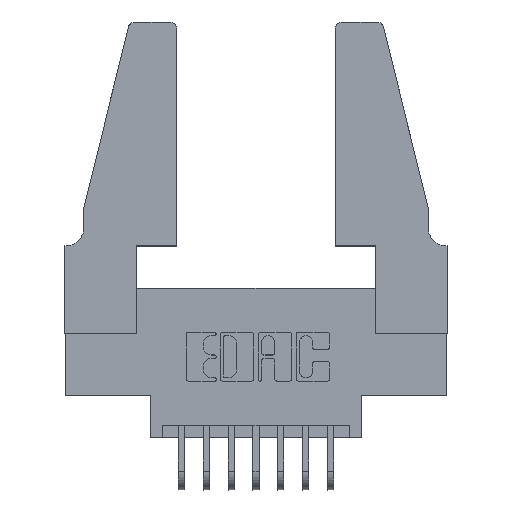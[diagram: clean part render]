
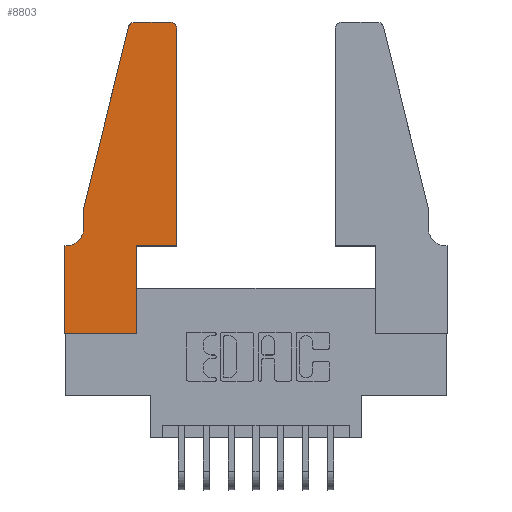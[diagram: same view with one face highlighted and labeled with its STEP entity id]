
A CAD part, top view. The second image highlights one B-rep face of the part: STEP entity #8803.
In plain terms, the highlighted planar face has unit normal (0, 0, 1).
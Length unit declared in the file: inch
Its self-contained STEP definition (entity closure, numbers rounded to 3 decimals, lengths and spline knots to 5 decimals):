
#18 = VECTOR ( 'NONE', #14092, 39.37008 ) ;
#74 = CARTESIAN_POINT ( 'NONE',  ( 0.284, 1.22, 0.37 ) ) ;
#455 = DIRECTION ( 'NONE',  ( 0., 0., 1. ) ) ;
#497 = LINE ( 'NONE', #12305, #11872 ) ;
#555 = CARTESIAN_POINT ( 'NONE',  ( 0.2865, 0., 0.37 ) ) ;
#579 = VERTEX_POINT ( 'NONE', #555 ) ;
#904 = EDGE_CURVE ( 'NONE', #11357, #10992, #4148, .T. ) ;
#951 = EDGE_CURVE ( 'NONE', #3013, #579, #11669, .T. ) ;
#1309 = DIRECTION ( 'NONE',  ( 1., 0., 0. ) ) ;
#1459 = CIRCLE ( 'NONE', #4887, 0.03 ) ;
#1518 = EDGE_CURVE ( 'NONE', #5218, #6235, #2289, .T. ) ;
#1893 = CARTESIAN_POINT ( 'NONE',  ( 0.4205, 1.25, 0.37 ) ) ;
#1919 = VECTOR ( 'NONE', #11491, 39.37008 ) ;
#2080 = CARTESIAN_POINT ( 'NONE',  ( 0.4505, 0.35, 0.37 ) ) ;
#2279 = DIRECTION ( 'NONE',  ( 0., 0., -1. ) ) ;
#2289 = LINE ( 'NONE', #10027, #1919 ) ;
#2444 = CARTESIAN_POINT ( 'NONE',  ( 0., 0.35, 0.37 ) ) ;
#2829 = DIRECTION ( 'NONE',  ( -0.239, -0.971, 0. ) ) ;
#2885 = LINE ( 'NONE', #7581, #8432 ) ;
#3013 = VERTEX_POINT ( 'NONE', #5641 ) ;
#3182 = LINE ( 'NONE', #4582, #18 ) ;
#3295 = VERTEX_POINT ( 'NONE', #8184 ) ;
#3577 = CARTESIAN_POINT ( 'NONE',  ( 0.2865, 0.35, 0.37 ) ) ;
#3605 = DIRECTION ( 'NONE',  ( 1., 0., 0. ) ) ;
#3645 = CARTESIAN_POINT ( 'NONE',  ( 0.0055, 0.35, 0.37 ) ) ;
#3731 = CARTESIAN_POINT ( 'NONE',  ( 0.25487, 1.22718, 0.37 ) ) ;
#4148 = LINE ( 'NONE', #2080, #6389 ) ;
#4316 = CARTESIAN_POINT ( 'NONE',  ( 0.4505, 0.35, 0.37 ) ) ;
#4422 = LINE ( 'NONE', #6341, #12572 ) ;
#4571 = CIRCLE ( 'NONE', #13946, 0.03 ) ;
#4582 = CARTESIAN_POINT ( 'NONE',  ( 0.2605, 1.25, 0.37 ) ) ;
#4646 = LINE ( 'NONE', #3577, #12780 ) ;
#4806 = VERTEX_POINT ( 'NONE', #9488 ) ;
#4812 = CARTESIAN_POINT ( 'NONE',  ( 0.284, 1.25, 0.37 ) ) ;
#4887 = AXIS2_PLACEMENT_3D ( 'NONE', #7293, #455, #8369 ) ;
#5198 = EDGE_CURVE ( 'NONE', #12901, #10067, #4571, .T. ) ;
#5206 = EDGE_LOOP ( 'NONE', ( #6011, #6132, #6167, #6295, #6393, #6473, #6546, #6568, #6668, #6693, #7019, #7049 ) ) ;
#5218 = VERTEX_POINT ( 'NONE', #3645 ) ;
#5641 = CARTESIAN_POINT ( 'NONE',  ( 0., 0., 0.37 ) ) ;
#5981 = EDGE_CURVE ( 'NONE', #10067, #7296, #497, .T. ) ;
#6011 = ORIENTED_EDGE ( 'NONE', *, *, #8704, .T. ) ;
#6132 = ORIENTED_EDGE ( 'NONE', *, *, #5198, .T. ) ;
#6134 = VERTEX_POINT ( 'NONE', #1893 ) ;
#6167 = ORIENTED_EDGE ( 'NONE', *, *, #5981, .T. ) ;
#6235 = VERTEX_POINT ( 'NONE', #11934 ) ;
#6295 = ORIENTED_EDGE ( 'NONE', *, *, #12556, .T. ) ;
#6341 = CARTESIAN_POINT ( 'NONE',  ( 0.4505, 0.35, 0.37 ) ) ;
#6389 = VECTOR ( 'NONE', #10767, 39.37008 ) ;
#6393 = ORIENTED_EDGE ( 'NONE', *, *, #6953, .T. ) ;
#6410 = CARTESIAN_POINT ( 'NONE',  ( 0., 0., 0.37 ) ) ;
#6473 = ORIENTED_EDGE ( 'NONE', *, *, #1518, .T. ) ;
#6546 = ORIENTED_EDGE ( 'NONE', *, *, #10330, .T. ) ;
#6568 = ORIENTED_EDGE ( 'NONE', *, *, #951, .T. ) ;
#6668 = ORIENTED_EDGE ( 'NONE', *, *, #8141, .T. ) ;
#6693 = ORIENTED_EDGE ( 'NONE', *, *, #9636, .T. ) ;
#6953 = EDGE_CURVE ( 'NONE', #4806, #5218, #13951, .T. ) ;
#7019 = ORIENTED_EDGE ( 'NONE', *, *, #904, .T. ) ;
#7049 = ORIENTED_EDGE ( 'NONE', *, *, #11183, .T. ) ;
#7293 = CARTESIAN_POINT ( 'NONE',  ( 0.4205, 1.22, 0.37 ) ) ;
#7296 = VERTEX_POINT ( 'NONE', #7425 ) ;
#7425 = CARTESIAN_POINT ( 'NONE',  ( 0.0755, 0.5, 0.37 ) ) ;
#7483 = LINE ( 'NONE', #6410, #12718 ) ;
#7581 = CARTESIAN_POINT ( 'NONE',  ( 0.0755, 0.5, 0.37 ) ) ;
#8031 = DIRECTION ( 'NONE',  ( 0., 0., 1. ) ) ;
#8037 = CARTESIAN_POINT ( 'NONE',  ( 0.4505, 1.22, 0.37 ) ) ;
#8141 = EDGE_CURVE ( 'NONE', #579, #3295, #4646, .T. ) ;
#8184 = CARTESIAN_POINT ( 'NONE',  ( 0.2865, 0.35, 0.37 ) ) ;
#8369 = DIRECTION ( 'NONE',  ( 1., 0., 0. ) ) ;
#8432 = VECTOR ( 'NONE', #13828, 39.37008 ) ;
#8524 = DIRECTION ( 'NONE',  ( 1., 0., 0. ) ) ;
#8567 = VECTOR ( 'NONE', #8524, 39.37008 ) ;
#8704 = EDGE_CURVE ( 'NONE', #6134, #12901, #3182, .T. ) ;
#8803 = ADVANCED_FACE ( 'NONE', ( #10488 ), #9067, .T. ) ;
#8914 = CARTESIAN_POINT ( 'NONE',  ( 0.0055, 0.42, 0.37 ) ) ;
#9067 = PLANE ( 'NONE',  #13638 ) ;
#9081 = DIRECTION ( 'NONE',  ( 0., 1., 0. ) ) ;
#9488 = CARTESIAN_POINT ( 'NONE',  ( 0.0755, 0.42, 0.37 ) ) ;
#9621 = AXIS2_PLACEMENT_3D ( 'NONE', #8914, #2279, #9970 ) ;
#9636 = EDGE_CURVE ( 'NONE', #3295, #11357, #4422, .T. ) ;
#9970 = DIRECTION ( 'NONE',  ( -1., 0., 0. ) ) ;
#10027 = CARTESIAN_POINT ( 'NONE',  ( 0.0755, 0.35, 0.37 ) ) ;
#10067 = VERTEX_POINT ( 'NONE', #3731 ) ;
#10109 = DIRECTION ( 'NONE',  ( 0., 0., 1. ) ) ;
#10330 = EDGE_CURVE ( 'NONE', #6235, #3013, #7483, .T. ) ;
#10488 = FACE_OUTER_BOUND ( 'NONE', #5206, .T. ) ;
#10767 = DIRECTION ( 'NONE',  ( 0., 1., 0. ) ) ;
#10992 = VERTEX_POINT ( 'NONE', #8037 ) ;
#11183 = EDGE_CURVE ( 'NONE', #10992, #6134, #1459, .T. ) ;
#11357 = VERTEX_POINT ( 'NONE', #4316 ) ;
#11491 = DIRECTION ( 'NONE',  ( -1., 0., 0. ) ) ;
#11669 = LINE ( 'NONE', #12026, #8567 ) ;
#11872 = VECTOR ( 'NONE', #2829, 39.37008 ) ;
#11934 = CARTESIAN_POINT ( 'NONE',  ( 0., 0.35, 0.37 ) ) ;
#12026 = CARTESIAN_POINT ( 'NONE',  ( 0., 0., 0.37 ) ) ;
#12305 = CARTESIAN_POINT ( 'NONE',  ( 0.0755, 0.5, 0.37 ) ) ;
#12556 = EDGE_CURVE ( 'NONE', #7296, #4806, #2885, .T. ) ;
#12572 = VECTOR ( 'NONE', #13679, 39.37008 ) ;
#12702 = DIRECTION ( 'NONE',  ( 0., -1., 0. ) ) ;
#12718 = VECTOR ( 'NONE', #12702, 39.37008 ) ;
#12780 = VECTOR ( 'NONE', #9081, 39.37008 ) ;
#12901 = VERTEX_POINT ( 'NONE', #4812 ) ;
#13638 = AXIS2_PLACEMENT_3D ( 'NONE', #2444, #10109, #3605 ) ;
#13679 = DIRECTION ( 'NONE',  ( 1., 0., 0. ) ) ;
#13828 = DIRECTION ( 'NONE',  ( 0., -1., 0. ) ) ;
#13946 = AXIS2_PLACEMENT_3D ( 'NONE', #74, #8031, #1309 ) ;
#13951 = CIRCLE ( 'NONE', #9621, 0.07 ) ;
#14092 = DIRECTION ( 'NONE',  ( -1., 0., 0. ) ) ;
